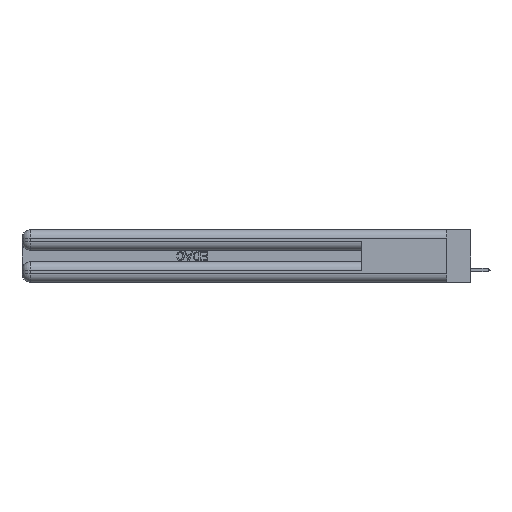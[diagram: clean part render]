
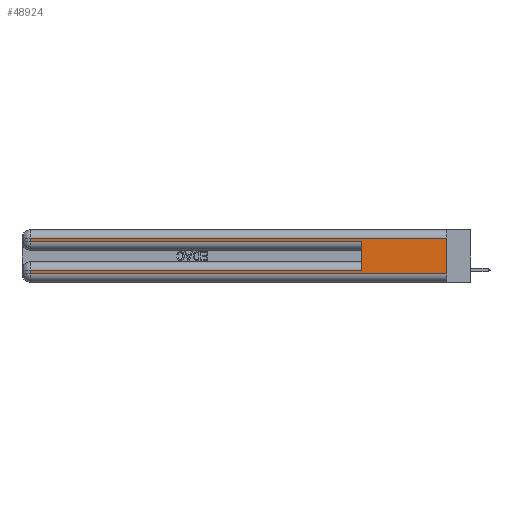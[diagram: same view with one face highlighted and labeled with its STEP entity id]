
A CAD part, left-side view. The second image highlights one B-rep face of the part: STEP entity #48924.
In plain terms, the highlighted planar face has unit normal (-1, 0, 0).
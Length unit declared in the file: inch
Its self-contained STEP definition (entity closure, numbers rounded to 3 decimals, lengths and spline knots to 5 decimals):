
#236 = LINE ( 'NONE', #50688, #5387 ) ;
#299 = CARTESIAN_POINT ( 'NONE',  ( 0., 2.94, 0.37 ) ) ;
#391 = VERTEX_POINT ( 'NONE', #7139 ) ;
#464 = LINE ( 'NONE', #14669, #29680 ) ;
#796 = DIRECTION ( 'NONE',  ( 0., 0., 1. ) ) ;
#1332 = EDGE_CURVE ( 'NONE', #16623, #28976, #30955, .T. ) ;
#3072 = PLANE ( 'NONE',  #49192 ) ;
#3214 = VERTEX_POINT ( 'NONE', #7134 ) ;
#3627 = ORIENTED_EDGE ( 'NONE', *, *, #50444, .T. ) ;
#4332 = EDGE_CURVE ( 'NONE', #3214, #23625, #51243, .T. ) ;
#4374 = FACE_OUTER_BOUND ( 'NONE', #5029, .T. ) ;
#5029 = EDGE_LOOP ( 'NONE', ( #21977, #35891, #17528, #3627, #22576, #37105, #49998, #8661 ) ) ;
#5387 = VECTOR ( 'NONE', #5484, 39.37008 ) ;
#5484 = DIRECTION ( 'NONE',  ( 0., -1., 0. ) ) ;
#7134 = CARTESIAN_POINT ( 'NONE',  ( 0., 2.94, 0.085 ) ) ;
#7139 = CARTESIAN_POINT ( 'NONE',  ( 0., 0., 0.06 ) ) ;
#7295 = EDGE_CURVE ( 'NONE', #12346, #3214, #464, .T. ) ;
#8661 = ORIENTED_EDGE ( 'NONE', *, *, #50881, .T. ) ;
#9128 = DIRECTION ( 'NONE',  ( 0., 1., 0. ) ) ;
#10398 = CARTESIAN_POINT ( 'NONE',  ( 0., 2.94, 0.31 ) ) ;
#10918 = VECTOR ( 'NONE', #796, 39.37008 ) ;
#11354 = CARTESIAN_POINT ( 'NONE',  ( 0., 0.6, 0.085 ) ) ;
#12250 = CARTESIAN_POINT ( 'NONE',  ( 0., 0., 0.06 ) ) ;
#12346 = VERTEX_POINT ( 'NONE', #11354 ) ;
#12413 = DIRECTION ( 'NONE',  ( 0., -1., 0. ) ) ;
#14221 = LINE ( 'NONE', #30111, #45951 ) ;
#14669 = CARTESIAN_POINT ( 'NONE',  ( 0., 0., 0.085 ) ) ;
#14983 = DIRECTION ( 'NONE',  ( 1., 0., 0. ) ) ;
#15975 = CARTESIAN_POINT ( 'NONE',  ( 0., 2.94, 0.285 ) ) ;
#16623 = VERTEX_POINT ( 'NONE', #10398 ) ;
#17528 = ORIENTED_EDGE ( 'NONE', *, *, #1332, .T. ) ;
#17886 = VECTOR ( 'NONE', #12413, 39.37008 ) ;
#18253 = VECTOR ( 'NONE', #39738, 39.37008 ) ;
#21839 = VERTEX_POINT ( 'NONE', #31029 ) ;
#21977 = ORIENTED_EDGE ( 'NONE', *, *, #33226, .F. ) ;
#22392 = LINE ( 'NONE', #12250, #17886 ) ;
#22576 = ORIENTED_EDGE ( 'NONE', *, *, #29155, .F. ) ;
#22596 = LINE ( 'NONE', #43300, #32500 ) ;
#23198 = DIRECTION ( 'NONE',  ( 0., 1., 0. ) ) ;
#23625 = VERTEX_POINT ( 'NONE', #31013 ) ;
#26372 = VECTOR ( 'NONE', #53409, 39.37008 ) ;
#28976 = VERTEX_POINT ( 'NONE', #15975 ) ;
#29155 = EDGE_CURVE ( 'NONE', #12346, #21839, #34833, .T. ) ;
#29680 = VECTOR ( 'NONE', #23198, 39.37008 ) ;
#30111 = CARTESIAN_POINT ( 'NONE',  ( 0., 0., 0.31 ) ) ;
#30955 = LINE ( 'NONE', #299, #26372 ) ;
#31013 = CARTESIAN_POINT ( 'NONE',  ( 0., 2.94, 0.06 ) ) ;
#31029 = CARTESIAN_POINT ( 'NONE',  ( 0., 0.6, 0.285 ) ) ;
#32500 = VECTOR ( 'NONE', #42937, 39.37008 ) ;
#33222 = EDGE_CURVE ( 'NONE', #51868, #16623, #14221, .T. ) ;
#33226 = EDGE_CURVE ( 'NONE', #51868, #391, #22596, .T. ) ;
#34833 = LINE ( 'NONE', #39546, #10918 ) ;
#35891 = ORIENTED_EDGE ( 'NONE', *, *, #33222, .T. ) ;
#37105 = ORIENTED_EDGE ( 'NONE', *, *, #7295, .T. ) ;
#39546 = CARTESIAN_POINT ( 'NONE',  ( 0., 0.6, 0.145 ) ) ;
#39738 = DIRECTION ( 'NONE',  ( 0., 0., -1. ) ) ;
#42937 = DIRECTION ( 'NONE',  ( 0., 0., -1. ) ) ;
#43300 = CARTESIAN_POINT ( 'NONE',  ( 0., 0., 0.37 ) ) ;
#43921 = DIRECTION ( 'NONE',  ( 0., 0., -1. ) ) ;
#45951 = VECTOR ( 'NONE', #9128, 39.37008 ) ;
#46692 = CARTESIAN_POINT ( 'NONE',  ( 0., 0., 0.31 ) ) ;
#47237 = CARTESIAN_POINT ( 'NONE',  ( 0., 2.94, 0.37 ) ) ;
#48924 = ADVANCED_FACE ( 'NONE', ( #4374 ), #3072, .F. ) ;
#49192 = AXIS2_PLACEMENT_3D ( 'NONE', #52988, #14983, #43921 ) ;
#49998 = ORIENTED_EDGE ( 'NONE', *, *, #4332, .T. ) ;
#50444 = EDGE_CURVE ( 'NONE', #28976, #21839, #236, .T. ) ;
#50688 = CARTESIAN_POINT ( 'NONE',  ( 0., 0., 0.285 ) ) ;
#50881 = EDGE_CURVE ( 'NONE', #23625, #391, #22392, .T. ) ;
#51243 = LINE ( 'NONE', #47237, #18253 ) ;
#51868 = VERTEX_POINT ( 'NONE', #46692 ) ;
#52988 = CARTESIAN_POINT ( 'NONE',  ( 0., 0., 0.37 ) ) ;
#53409 = DIRECTION ( 'NONE',  ( 0., 0., -1. ) ) ;
